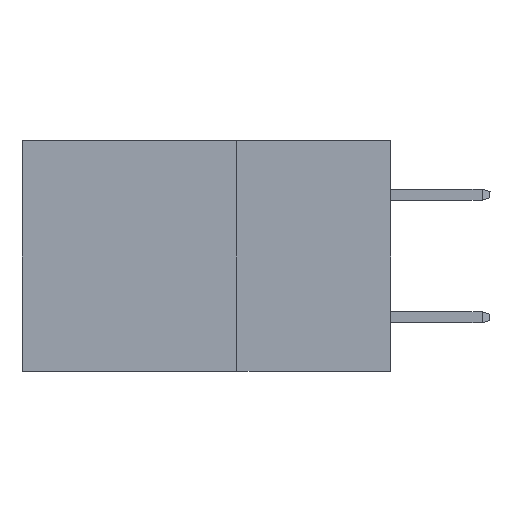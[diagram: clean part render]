
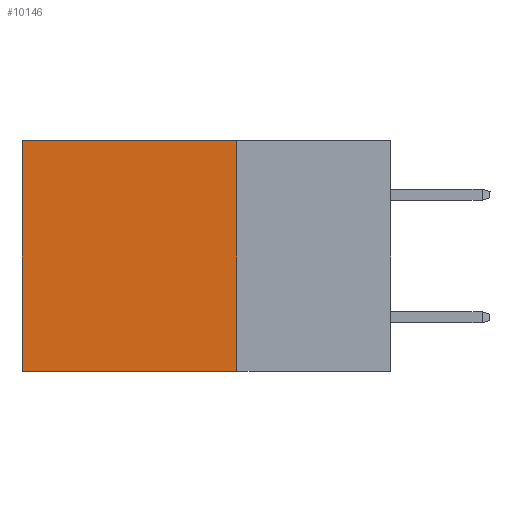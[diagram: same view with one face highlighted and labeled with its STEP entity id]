
A CAD part, left-side view. The second image highlights one B-rep face of the part: STEP entity #10146.
In plain terms, the highlighted planar face has unit normal (-1, 0, 0).
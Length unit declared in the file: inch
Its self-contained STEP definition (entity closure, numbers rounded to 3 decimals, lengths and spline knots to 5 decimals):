
#443 = DIRECTION ( 'NONE',  ( 0., 0., -1. ) ) ;
#927 = AXIS2_PLACEMENT_3D ( 'NONE', #11733, #10692, #1166 ) ;
#1166 = DIRECTION ( 'NONE',  ( 0., 0., -1. ) ) ;
#1510 = DIRECTION ( 'NONE',  ( 0., 0., -1. ) ) ;
#1577 = VERTEX_POINT ( 'NONE', #11041 ) ;
#1658 = EDGE_CURVE ( 'NONE', #10531, #3086, #8886, .T. ) ;
#1975 = VERTEX_POINT ( 'NONE', #12693 ) ;
#2126 = VECTOR ( 'NONE', #1510, 39.37008 ) ;
#2398 = LINE ( 'NONE', #4351, #10278 ) ;
#3086 = VERTEX_POINT ( 'NONE', #10215 ) ;
#3192 = ORIENTED_EDGE ( 'NONE', *, *, #13590, .F. ) ;
#3294 = VECTOR ( 'NONE', #13651, 39.37008 ) ;
#4228 = FACE_OUTER_BOUND ( 'NONE', #7107, .T. ) ;
#4351 = CARTESIAN_POINT ( 'NONE',  ( 0.2875, 0.25, 0. ) ) ;
#6120 = CARTESIAN_POINT ( 'NONE',  ( 0.2875, 0.25, -0.375 ) ) ;
#6561 = LINE ( 'NONE', #9969, #12219 ) ;
#6641 = DIRECTION ( 'NONE',  ( 0., 1., 0. ) ) ;
#6690 = PLANE ( 'NONE',  #927 ) ;
#7107 = EDGE_LOOP ( 'NONE', ( #7486, #3192, #8602, #12895 ) ) ;
#7486 = ORIENTED_EDGE ( 'NONE', *, *, #1658, .T. ) ;
#8602 = ORIENTED_EDGE ( 'NONE', *, *, #8894, .F. ) ;
#8886 = LINE ( 'NONE', #10973, #2126 ) ;
#8894 = EDGE_CURVE ( 'NONE', #1577, #1975, #6561, .T. ) ;
#9969 = CARTESIAN_POINT ( 'NONE',  ( 0.2875, 0.25, -0.375 ) ) ;
#10146 = ADVANCED_FACE ( 'NONE', ( #4228 ), #6690, .F. ) ;
#10215 = CARTESIAN_POINT ( 'NONE',  ( 0.2875, 0.6, -0.375 ) ) ;
#10278 = VECTOR ( 'NONE', #6641, 39.37008 ) ;
#10531 = VERTEX_POINT ( 'NONE', #12763 ) ;
#10692 = DIRECTION ( 'NONE',  ( 1., 0., 0. ) ) ;
#10973 = CARTESIAN_POINT ( 'NONE',  ( 0.2875, 0.6, -0.375 ) ) ;
#11041 = CARTESIAN_POINT ( 'NONE',  ( 0.2875, 0.25, 0. ) ) ;
#11733 = CARTESIAN_POINT ( 'NONE',  ( 0.2875, 0.25, -0.375 ) ) ;
#11836 = EDGE_CURVE ( 'NONE', #1577, #10531, #2398, .T. ) ;
#12219 = VECTOR ( 'NONE', #443, 39.37008 ) ;
#12591 = LINE ( 'NONE', #6120, #3294 ) ;
#12693 = CARTESIAN_POINT ( 'NONE',  ( 0.2875, 0.25, -0.375 ) ) ;
#12763 = CARTESIAN_POINT ( 'NONE',  ( 0.2875, 0.6, 0. ) ) ;
#12895 = ORIENTED_EDGE ( 'NONE', *, *, #11836, .T. ) ;
#13590 = EDGE_CURVE ( 'NONE', #1975, #3086, #12591, .T. ) ;
#13651 = DIRECTION ( 'NONE',  ( 0., 1., 0. ) ) ;
